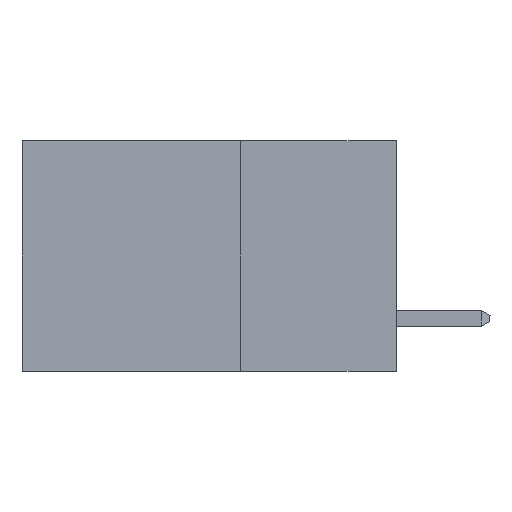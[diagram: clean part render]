
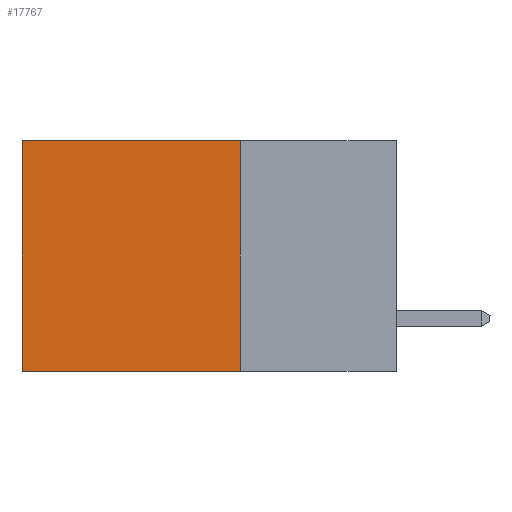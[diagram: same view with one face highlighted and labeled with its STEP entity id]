
A CAD part, left-side view. The second image highlights one B-rep face of the part: STEP entity #17767.
In plain terms, the highlighted planar face has unit normal (-1, 0, 0).
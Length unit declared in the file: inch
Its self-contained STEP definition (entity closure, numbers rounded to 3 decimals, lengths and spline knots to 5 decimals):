
#621 = ORIENTED_EDGE ( 'NONE', *, *, #10811, .T. ) ;
#998 = CARTESIAN_POINT ( 'NONE',  ( 0.298, 0.25, -0.37 ) ) ;
#1171 = CARTESIAN_POINT ( 'NONE',  ( 0.298, 0.6, 0. ) ) ;
#1212 = ORIENTED_EDGE ( 'NONE', *, *, #11054, .F. ) ;
#1712 = CARTESIAN_POINT ( 'NONE',  ( 0.298, 0.25, 0. ) ) ;
#2802 = LINE ( 'NONE', #11610, #10818 ) ;
#3054 = LINE ( 'NONE', #1171, #6861 ) ;
#3327 = DIRECTION ( 'NONE',  ( 0., 1., 0. ) ) ;
#4200 = VERTEX_POINT ( 'NONE', #998 ) ;
#4216 = ORIENTED_EDGE ( 'NONE', *, *, #16081, .F. ) ;
#4980 = VERTEX_POINT ( 'NONE', #16054 ) ;
#5472 = EDGE_CURVE ( 'NONE', #14852, #5709, #5725, .T. ) ;
#5709 = VERTEX_POINT ( 'NONE', #14179 ) ;
#5725 = LINE ( 'NONE', #20318, #20035 ) ;
#6301 = AXIS2_PLACEMENT_3D ( 'NONE', #1712, #8106, #17896 ) ;
#6861 = VECTOR ( 'NONE', #18894, 39.37008 ) ;
#7513 = VECTOR ( 'NONE', #11695, 39.37008 ) ;
#8106 = DIRECTION ( 'NONE',  ( 1., 0., 0. ) ) ;
#8221 = FACE_OUTER_BOUND ( 'NONE', #18977, .T. ) ;
#10811 = EDGE_CURVE ( 'NONE', #5709, #4980, #3054, .T. ) ;
#10818 = VECTOR ( 'NONE', #17862, 39.37008 ) ;
#11054 = EDGE_CURVE ( 'NONE', #14852, #4200, #2802, .T. ) ;
#11610 = CARTESIAN_POINT ( 'NONE',  ( 0.298, 0.25, 0. ) ) ;
#11695 = DIRECTION ( 'NONE',  ( 0., 1., 0. ) ) ;
#13526 = ORIENTED_EDGE ( 'NONE', *, *, #5472, .T. ) ;
#14083 = CARTESIAN_POINT ( 'NONE',  ( 0.298, 0.25, 0. ) ) ;
#14179 = CARTESIAN_POINT ( 'NONE',  ( 0.298, 0.6, 0. ) ) ;
#14852 = VERTEX_POINT ( 'NONE', #14083 ) ;
#15052 = CARTESIAN_POINT ( 'NONE',  ( 0.298, 0.25, -0.37 ) ) ;
#16054 = CARTESIAN_POINT ( 'NONE',  ( 0.298, 0.6, -0.37 ) ) ;
#16081 = EDGE_CURVE ( 'NONE', #4200, #4980, #20065, .T. ) ;
#16214 = PLANE ( 'NONE',  #6301 ) ;
#17767 = ADVANCED_FACE ( 'NONE', ( #8221 ), #16214, .F. ) ;
#17862 = DIRECTION ( 'NONE',  ( 0., 0., -1. ) ) ;
#17896 = DIRECTION ( 'NONE',  ( 0., 0., -1. ) ) ;
#18894 = DIRECTION ( 'NONE',  ( 0., 0., -1. ) ) ;
#18977 = EDGE_LOOP ( 'NONE', ( #621, #4216, #1212, #13526 ) ) ;
#20035 = VECTOR ( 'NONE', #3327, 39.37008 ) ;
#20065 = LINE ( 'NONE', #15052, #7513 ) ;
#20318 = CARTESIAN_POINT ( 'NONE',  ( 0.298, 0.25, 0. ) ) ;
